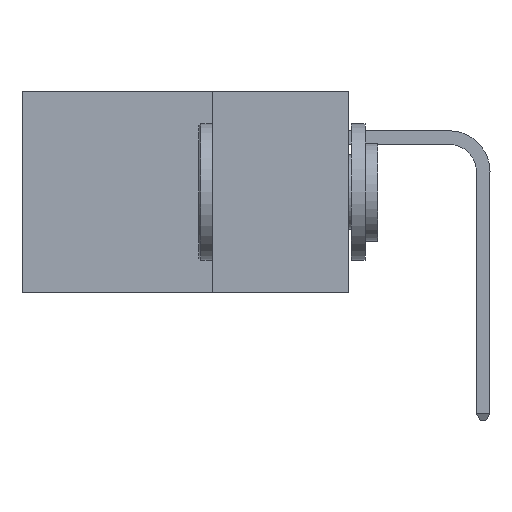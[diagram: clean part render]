
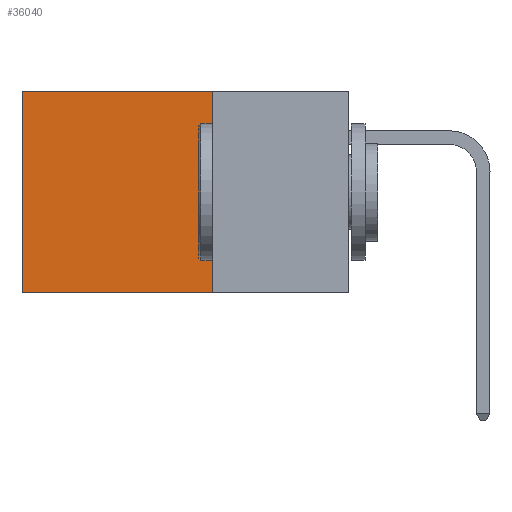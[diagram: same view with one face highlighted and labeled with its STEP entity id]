
A CAD part, left-side view. The second image highlights one B-rep face of the part: STEP entity #36040.
In plain terms, the highlighted planar face has unit normal (-1, 0, 0).
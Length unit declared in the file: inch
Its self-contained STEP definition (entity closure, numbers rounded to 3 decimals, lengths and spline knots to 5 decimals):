
#183 = VERTEX_POINT ( 'NONE', #21505 ) ;
#301 = ORIENTED_EDGE ( 'NONE', *, *, #33374, .T. ) ;
#1305 = VECTOR ( 'NONE', #4367, 39.37008 ) ;
#1408 = CARTESIAN_POINT ( 'NONE',  ( 0.2875, 0.25, 0. ) ) ;
#2239 = LINE ( 'NONE', #1408, #1305 ) ;
#3792 = VERTEX_POINT ( 'NONE', #34816 ) ;
#4367 = DIRECTION ( 'NONE',  ( 0., 1., 0. ) ) ;
#4370 = ORIENTED_EDGE ( 'NONE', *, *, #10531, .T. ) ;
#4654 = EDGE_LOOP ( 'NONE', ( #4370, #25501, #31420, #301 ) ) ;
#6199 = CARTESIAN_POINT ( 'NONE',  ( 0.2875, 0.6, 0. ) ) ;
#6728 = CARTESIAN_POINT ( 'NONE',  ( 0.2875, 0.25, -0.37 ) ) ;
#9455 = VERTEX_POINT ( 'NONE', #24499 ) ;
#10531 = EDGE_CURVE ( 'NONE', #15343, #9455, #21538, .T. ) ;
#10536 = DIRECTION ( 'NONE',  ( 1., 0., 0. ) ) ;
#14221 = DIRECTION ( 'NONE',  ( 0., 0., -1. ) ) ;
#15343 = VERTEX_POINT ( 'NONE', #6199 ) ;
#17542 = LINE ( 'NONE', #22800, #24365 ) ;
#17811 = DIRECTION ( 'NONE',  ( 0., 0., -1. ) ) ;
#19090 = PLANE ( 'NONE',  #24012 ) ;
#21505 = CARTESIAN_POINT ( 'NONE',  ( 0.2875, 0.25, -0.37 ) ) ;
#21538 = LINE ( 'NONE', #32051, #36582 ) ;
#22341 = VECTOR ( 'NONE', #26935, 39.37008 ) ;
#22800 = CARTESIAN_POINT ( 'NONE',  ( 0.2875, 0.25, 0. ) ) ;
#24012 = AXIS2_PLACEMENT_3D ( 'NONE', #27798, #10536, #30609 ) ;
#24365 = VECTOR ( 'NONE', #14221, 39.37008 ) ;
#24499 = CARTESIAN_POINT ( 'NONE',  ( 0.2875, 0.6, -0.37 ) ) ;
#24986 = EDGE_CURVE ( 'NONE', #3792, #183, #17542, .T. ) ;
#25266 = FACE_OUTER_BOUND ( 'NONE', #4654, .T. ) ;
#25501 = ORIENTED_EDGE ( 'NONE', *, *, #27101, .F. ) ;
#26935 = DIRECTION ( 'NONE',  ( 0., 1., 0. ) ) ;
#27101 = EDGE_CURVE ( 'NONE', #183, #9455, #29942, .T. ) ;
#27798 = CARTESIAN_POINT ( 'NONE',  ( 0.2875, 0.25, 0. ) ) ;
#29942 = LINE ( 'NONE', #6728, #22341 ) ;
#30609 = DIRECTION ( 'NONE',  ( 0., 0., -1. ) ) ;
#31420 = ORIENTED_EDGE ( 'NONE', *, *, #24986, .F. ) ;
#32051 = CARTESIAN_POINT ( 'NONE',  ( 0.2875, 0.6, 0. ) ) ;
#33374 = EDGE_CURVE ( 'NONE', #3792, #15343, #2239, .T. ) ;
#34816 = CARTESIAN_POINT ( 'NONE',  ( 0.2875, 0.25, 0. ) ) ;
#36040 = ADVANCED_FACE ( 'NONE', ( #25266 ), #19090, .F. ) ;
#36582 = VECTOR ( 'NONE', #17811, 39.37008 ) ;
